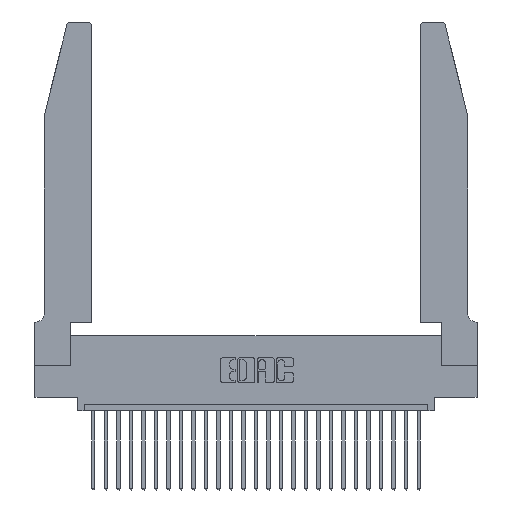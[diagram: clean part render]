
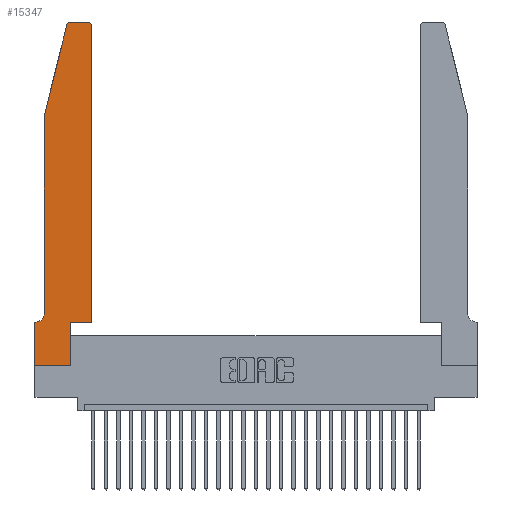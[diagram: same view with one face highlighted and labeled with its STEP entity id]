
A CAD part, top view. The second image highlights one B-rep face of the part: STEP entity #15347.
In plain terms, the highlighted planar face has unit normal (0, 0, 1).
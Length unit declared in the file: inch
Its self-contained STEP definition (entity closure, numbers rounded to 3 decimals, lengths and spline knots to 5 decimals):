
#209 = DIRECTION ( 'NONE',  ( -1., 0., 0. ) ) ;
#352 = CIRCLE ( 'NONE', #1606, 0.03 ) ;
#1083 = VERTEX_POINT ( 'NONE', #10623 ) ;
#1360 = DIRECTION ( 'NONE',  ( -1., 0., 0. ) ) ;
#1606 = AXIS2_PLACEMENT_3D ( 'NONE', #25713, #17328, #8941 ) ;
#1662 = AXIS2_PLACEMENT_3D ( 'NONE', #3693, #7999, #9848 ) ;
#2399 = DIRECTION ( 'NONE',  ( -1., 0., 0. ) ) ;
#2548 = CARTESIAN_POINT ( 'NONE',  ( 0.4505, 0.35, 0.37 ) ) ;
#2630 = VERTEX_POINT ( 'NONE', #7129 ) ;
#2634 = LINE ( 'NONE', #12903, #13497 ) ;
#2709 = CARTESIAN_POINT ( 'NONE',  ( 0.2865, 0., 0.37 ) ) ;
#3105 = EDGE_CURVE ( 'NONE', #21371, #20108, #3762, .T. ) ;
#3291 = LINE ( 'NONE', #5870, #7582 ) ;
#3693 = CARTESIAN_POINT ( 'NONE',  ( 0., 0.35, 0.37 ) ) ;
#3762 = CIRCLE ( 'NONE', #20418, 0.07 ) ;
#4845 = EDGE_CURVE ( 'NONE', #14632, #21371, #24739, .T. ) ;
#4909 = CARTESIAN_POINT ( 'NONE',  ( 0.0055, 0.35, 0.37 ) ) ;
#5104 = DIRECTION ( 'NONE',  ( -0.239, -0.971, 0. ) ) ;
#5151 = DIRECTION ( 'NONE',  ( 0., 1., 0. ) ) ;
#5364 = EDGE_CURVE ( 'NONE', #9774, #12890, #2634, .T. ) ;
#5442 = VERTEX_POINT ( 'NONE', #2709 ) ;
#5530 = CARTESIAN_POINT ( 'NONE',  ( 0., 0., 0.37 ) ) ;
#5870 = CARTESIAN_POINT ( 'NONE',  ( 0.4505, 0.35, 0.37 ) ) ;
#6312 = VERTEX_POINT ( 'NONE', #22577 ) ;
#6471 = CARTESIAN_POINT ( 'NONE',  ( 0., 0.35, 0.37 ) ) ;
#6478 = DIRECTION ( 'NONE',  ( 0., -1., 0. ) ) ;
#7129 = CARTESIAN_POINT ( 'NONE',  ( 0.4205, 2.75, 0.37 ) ) ;
#7572 = ORIENTED_EDGE ( 'NONE', *, *, #9957, .T. ) ;
#7582 = VECTOR ( 'NONE', #16442, 39.37008 ) ;
#7684 = ORIENTED_EDGE ( 'NONE', *, *, #3105, .T. ) ;
#7999 = DIRECTION ( 'NONE',  ( 0., 0., 1. ) ) ;
#8197 = ORIENTED_EDGE ( 'NONE', *, *, #24770, .T. ) ;
#8256 = VECTOR ( 'NONE', #2399, 39.37008 ) ;
#8941 = DIRECTION ( 'NONE',  ( 1., 0., 0. ) ) ;
#8992 = LINE ( 'NONE', #19566, #10656 ) ;
#9082 = VERTEX_POINT ( 'NONE', #20163 ) ;
#9215 = EDGE_CURVE ( 'NONE', #18950, #2630, #10042, .T. ) ;
#9774 = VERTEX_POINT ( 'NONE', #6471 ) ;
#9848 = DIRECTION ( 'NONE',  ( 1., 0., 0. ) ) ;
#9957 = EDGE_CURVE ( 'NONE', #20465, #14632, #13583, .T. ) ;
#10028 = EDGE_CURVE ( 'NONE', #12890, #5442, #8992, .T. ) ;
#10042 = CIRCLE ( 'NONE', #17886, 0.03 ) ;
#10623 = CARTESIAN_POINT ( 'NONE',  ( 0.2865, 0.35, 0.37 ) ) ;
#10656 = VECTOR ( 'NONE', #19921, 39.37008 ) ;
#10726 = ORIENTED_EDGE ( 'NONE', *, *, #10028, .T. ) ;
#10742 = CARTESIAN_POINT ( 'NONE',  ( 0.0755, 2., 0.37 ) ) ;
#10905 = LINE ( 'NONE', #23638, #8256 ) ;
#11439 = CARTESIAN_POINT ( 'NONE',  ( 0.2865, 0.35, 0.37 ) ) ;
#12417 = ORIENTED_EDGE ( 'NONE', *, *, #24504, .T. ) ;
#12506 = CARTESIAN_POINT ( 'NONE',  ( 0.25487, 2.72718, 0.37 ) ) ;
#12890 = VERTEX_POINT ( 'NONE', #5530 ) ;
#12903 = CARTESIAN_POINT ( 'NONE',  ( 0., 0., 0.37 ) ) ;
#13497 = VECTOR ( 'NONE', #6478, 39.37008 ) ;
#13583 = LINE ( 'NONE', #21801, #19191 ) ;
#13779 = ORIENTED_EDGE ( 'NONE', *, *, #13871, .T. ) ;
#13862 = VECTOR ( 'NONE', #21998, 39.37008 ) ;
#13871 = EDGE_CURVE ( 'NONE', #6312, #20465, #352, .T. ) ;
#13929 = DIRECTION ( 'NONE',  ( 0., 0., -1. ) ) ;
#14632 = VERTEX_POINT ( 'NONE', #10742 ) ;
#14998 = CARTESIAN_POINT ( 'NONE',  ( 0.0755, 0.35, 0.37 ) ) ;
#15347 = ADVANCED_FACE ( 'NONE', ( #24382 ), #26774, .T. ) ;
#16442 = DIRECTION ( 'NONE',  ( 1., 0., 0. ) ) ;
#17328 = DIRECTION ( 'NONE',  ( 0., 0., 1. ) ) ;
#17365 = ORIENTED_EDGE ( 'NONE', *, *, #23014, .T. ) ;
#17883 = EDGE_LOOP ( 'NONE', ( #8197, #13779, #7572, #23354, #7684, #17981, #18855, #10726, #17365, #12417, #20355, #26020 ) ) ;
#17886 = AXIS2_PLACEMENT_3D ( 'NONE', #26907, #25096, #18541 ) ;
#17981 = ORIENTED_EDGE ( 'NONE', *, *, #19289, .T. ) ;
#18342 = CARTESIAN_POINT ( 'NONE',  ( 0.0755, 0.42, 0.37 ) ) ;
#18533 = VECTOR ( 'NONE', #5151, 39.37008 ) ;
#18541 = DIRECTION ( 'NONE',  ( 1., 0., 0. ) ) ;
#18855 = ORIENTED_EDGE ( 'NONE', *, *, #5364, .T. ) ;
#18950 = VERTEX_POINT ( 'NONE', #19642 ) ;
#19191 = VECTOR ( 'NONE', #5104, 39.37008 ) ;
#19289 = EDGE_CURVE ( 'NONE', #20108, #9774, #27110, .T. ) ;
#19566 = CARTESIAN_POINT ( 'NONE',  ( 0., 0., 0.37 ) ) ;
#19642 = CARTESIAN_POINT ( 'NONE',  ( 0.4505, 2.72, 0.37 ) ) ;
#19815 = VECTOR ( 'NONE', #209, 39.37008 ) ;
#19921 = DIRECTION ( 'NONE',  ( 1., 0., 0. ) ) ;
#20108 = VERTEX_POINT ( 'NONE', #4909 ) ;
#20163 = CARTESIAN_POINT ( 'NONE',  ( 0.4505, 0.35, 0.37 ) ) ;
#20355 = ORIENTED_EDGE ( 'NONE', *, *, #22911, .T. ) ;
#20418 = AXIS2_PLACEMENT_3D ( 'NONE', #26815, #13929, #1360 ) ;
#20465 = VERTEX_POINT ( 'NONE', #12506 ) ;
#21371 = VERTEX_POINT ( 'NONE', #18342 ) ;
#21801 = CARTESIAN_POINT ( 'NONE',  ( 0.0755, 2., 0.37 ) ) ;
#21998 = DIRECTION ( 'NONE',  ( 0., -1., 0. ) ) ;
#22185 = CARTESIAN_POINT ( 'NONE',  ( 0.0755, 2., 0.37 ) ) ;
#22577 = CARTESIAN_POINT ( 'NONE',  ( 0.284, 2.75, 0.37 ) ) ;
#22911 = EDGE_CURVE ( 'NONE', #9082, #18950, #25469, .T. ) ;
#23014 = EDGE_CURVE ( 'NONE', #5442, #1083, #24800, .T. ) ;
#23354 = ORIENTED_EDGE ( 'NONE', *, *, #4845, .T. ) ;
#23448 = DIRECTION ( 'NONE',  ( 0., 1., 0. ) ) ;
#23638 = CARTESIAN_POINT ( 'NONE',  ( 0.2605, 2.75, 0.37 ) ) ;
#24382 = FACE_OUTER_BOUND ( 'NONE', #17883, .T. ) ;
#24504 = EDGE_CURVE ( 'NONE', #1083, #9082, #3291, .T. ) ;
#24739 = LINE ( 'NONE', #22185, #13862 ) ;
#24770 = EDGE_CURVE ( 'NONE', #2630, #6312, #10905, .T. ) ;
#24800 = LINE ( 'NONE', #11439, #18533 ) ;
#25096 = DIRECTION ( 'NONE',  ( 0., 0., 1. ) ) ;
#25469 = LINE ( 'NONE', #2548, #27084 ) ;
#25713 = CARTESIAN_POINT ( 'NONE',  ( 0.284, 2.72, 0.37 ) ) ;
#26020 = ORIENTED_EDGE ( 'NONE', *, *, #9215, .T. ) ;
#26774 = PLANE ( 'NONE',  #1662 ) ;
#26815 = CARTESIAN_POINT ( 'NONE',  ( 0.0055, 0.42, 0.37 ) ) ;
#26907 = CARTESIAN_POINT ( 'NONE',  ( 0.4205, 2.72, 0.37 ) ) ;
#27084 = VECTOR ( 'NONE', #23448, 39.37008 ) ;
#27110 = LINE ( 'NONE', #14998, #19815 ) ;
